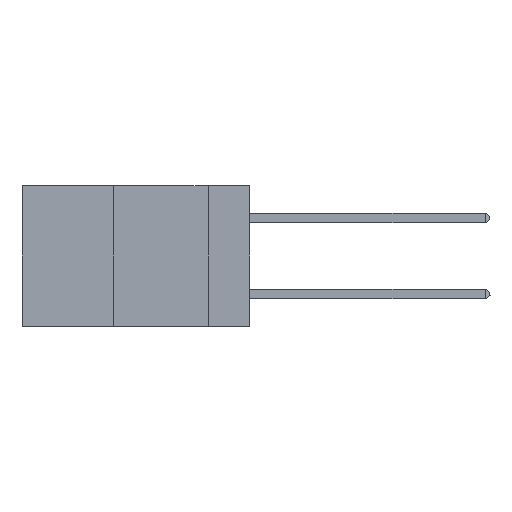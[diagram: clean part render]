
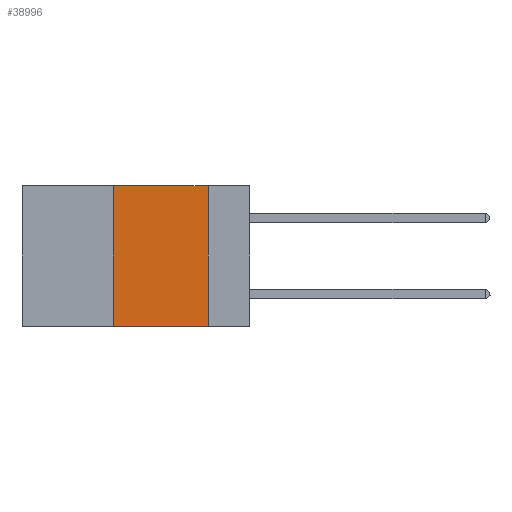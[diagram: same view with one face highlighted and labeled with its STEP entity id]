
A CAD part, left-side view. The second image highlights one B-rep face of the part: STEP entity #38996.
In plain terms, the highlighted planar face has unit normal (-1, 0, 0).
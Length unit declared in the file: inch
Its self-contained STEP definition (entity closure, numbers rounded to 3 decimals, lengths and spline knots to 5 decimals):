
#88 = CARTESIAN_POINT ( 'NONE',  ( 0., 0.6, -0.37 ) ) ;
#283 = LINE ( 'NONE', #27655, #7914 ) ;
#691 = CARTESIAN_POINT ( 'NONE',  ( 0., 0.36, 0. ) ) ;
#1479 = VERTEX_POINT ( 'NONE', #31198 ) ;
#2569 = FACE_OUTER_BOUND ( 'NONE', #27629, .T. ) ;
#3135 = PLANE ( 'NONE',  #15845 ) ;
#3218 = CARTESIAN_POINT ( 'NONE',  ( 0., 0.36, 0. ) ) ;
#3787 = CARTESIAN_POINT ( 'NONE',  ( 0., 0.6, 0. ) ) ;
#7083 = DIRECTION ( 'NONE',  ( 0., -1., 0. ) ) ;
#7914 = VECTOR ( 'NONE', #11893, 39.37008 ) ;
#8932 = LINE ( 'NONE', #3218, #24726 ) ;
#11826 = LINE ( 'NONE', #88, #34050 ) ;
#11893 = DIRECTION ( 'NONE',  ( 0., 0., -1. ) ) ;
#12490 = EDGE_CURVE ( 'NONE', #1479, #28494, #8932, .T. ) ;
#14397 = LINE ( 'NONE', #3787, #38479 ) ;
#15845 = AXIS2_PLACEMENT_3D ( 'NONE', #34830, #15928, #37914 ) ;
#15916 = ORIENTED_EDGE ( 'NONE', *, *, #34964, .F. ) ;
#15928 = DIRECTION ( 'NONE',  ( 1., 0., 0. ) ) ;
#17722 = EDGE_CURVE ( 'NONE', #1479, #24708, #11826, .T. ) ;
#23061 = VERTEX_POINT ( 'NONE', #36101 ) ;
#24708 = VERTEX_POINT ( 'NONE', #29152 ) ;
#24726 = VECTOR ( 'NONE', #31768, 39.37008 ) ;
#27629 = EDGE_LOOP ( 'NONE', ( #34686, #15916, #39977, #38035 ) ) ;
#27655 = CARTESIAN_POINT ( 'NONE',  ( 0., 0.11, 0. ) ) ;
#28494 = VERTEX_POINT ( 'NONE', #691 ) ;
#28610 = DIRECTION ( 'NONE',  ( 0., -1., 0. ) ) ;
#29152 = CARTESIAN_POINT ( 'NONE',  ( 0., 0.11, -0.37 ) ) ;
#30712 = EDGE_CURVE ( 'NONE', #23061, #24708, #283, .T. ) ;
#31198 = CARTESIAN_POINT ( 'NONE',  ( 0., 0.36, -0.37 ) ) ;
#31768 = DIRECTION ( 'NONE',  ( 0., 0., 1. ) ) ;
#34050 = VECTOR ( 'NONE', #28610, 39.37008 ) ;
#34686 = ORIENTED_EDGE ( 'NONE', *, *, #30712, .F. ) ;
#34830 = CARTESIAN_POINT ( 'NONE',  ( 0., 0.6, 0. ) ) ;
#34964 = EDGE_CURVE ( 'NONE', #28494, #23061, #14397, .T. ) ;
#36101 = CARTESIAN_POINT ( 'NONE',  ( 0., 0.11, 0. ) ) ;
#37914 = DIRECTION ( 'NONE',  ( 0., 0., -1. ) ) ;
#38035 = ORIENTED_EDGE ( 'NONE', *, *, #17722, .T. ) ;
#38479 = VECTOR ( 'NONE', #7083, 39.37008 ) ;
#38996 = ADVANCED_FACE ( 'NONE', ( #2569 ), #3135, .F. ) ;
#39977 = ORIENTED_EDGE ( 'NONE', *, *, #12490, .F. ) ;
